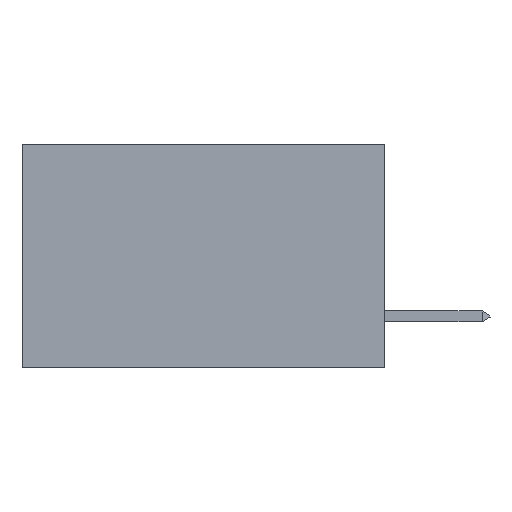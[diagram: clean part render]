
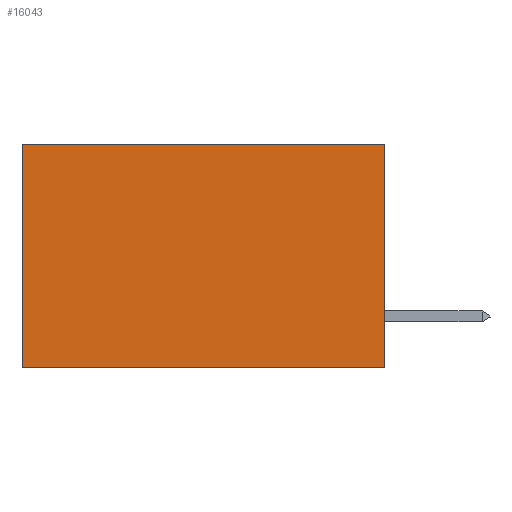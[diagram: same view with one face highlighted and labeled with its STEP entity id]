
A CAD part, left-side view. The second image highlights one B-rep face of the part: STEP entity #16043.
In plain terms, the highlighted planar face has unit normal (-1, 0, 0).
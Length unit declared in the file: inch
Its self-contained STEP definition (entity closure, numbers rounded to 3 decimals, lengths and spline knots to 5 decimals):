
#561 = EDGE_CURVE ( 'NONE', #37668, #39384, #48474, .T. ) ;
#1286 = DIRECTION ( 'NONE',  ( 0., 0., -1. ) ) ;
#5961 = CARTESIAN_POINT ( 'NONE',  ( 0.2875, 0., 0. ) ) ;
#7498 = VECTOR ( 'NONE', #41490, 39.37008 ) ;
#7872 = AXIS2_PLACEMENT_3D ( 'NONE', #12150, #24251, #1286 ) ;
#9865 = EDGE_CURVE ( 'NONE', #48452, #37668, #19689, .T. ) ;
#12098 = DIRECTION ( 'NONE',  ( 0., 1., 0. ) ) ;
#12150 = CARTESIAN_POINT ( 'NONE',  ( 0.2875, 0., 0. ) ) ;
#12496 = VECTOR ( 'NONE', #34595, 39.37008 ) ;
#13403 = DIRECTION ( 'NONE',  ( 0., 0., -1. ) ) ;
#13485 = EDGE_CURVE ( 'NONE', #48452, #42538, #37122, .T. ) ;
#14291 = VECTOR ( 'NONE', #13403, 39.37008 ) ;
#15569 = CARTESIAN_POINT ( 'NONE',  ( 0.2875, 0., 0. ) ) ;
#16043 = ADVANCED_FACE ( 'NONE', ( #45341 ), #35200, .F. ) ;
#18028 = ORIENTED_EDGE ( 'NONE', *, *, #24321, .T. ) ;
#18927 = CARTESIAN_POINT ( 'NONE',  ( 0.2875, 0.6, 0. ) ) ;
#19689 = LINE ( 'NONE', #5961, #14291 ) ;
#24251 = DIRECTION ( 'NONE',  ( 1., 0., 0. ) ) ;
#24321 = EDGE_CURVE ( 'NONE', #42538, #39384, #42543, .T. ) ;
#26009 = ORIENTED_EDGE ( 'NONE', *, *, #13485, .T. ) ;
#26875 = VECTOR ( 'NONE', #12098, 39.37008 ) ;
#29917 = CARTESIAN_POINT ( 'NONE',  ( 0.2875, 0., -0.37 ) ) ;
#30048 = ORIENTED_EDGE ( 'NONE', *, *, #561, .F. ) ;
#31444 = CARTESIAN_POINT ( 'NONE',  ( 0.2875, 0., 0. ) ) ;
#34595 = DIRECTION ( 'NONE',  ( 0., 0., -1. ) ) ;
#35200 = PLANE ( 'NONE',  #7872 ) ;
#36214 = CARTESIAN_POINT ( 'NONE',  ( 0.2875, 0.6, -0.37 ) ) ;
#36752 = EDGE_LOOP ( 'NONE', ( #18028, #30048, #45795, #26009 ) ) ;
#37122 = LINE ( 'NONE', #31444, #26875 ) ;
#37127 = CARTESIAN_POINT ( 'NONE',  ( 0.2875, 0., -0.37 ) ) ;
#37272 = CARTESIAN_POINT ( 'NONE',  ( 0.2875, 0.6, 0. ) ) ;
#37668 = VERTEX_POINT ( 'NONE', #29917 ) ;
#39384 = VERTEX_POINT ( 'NONE', #36214 ) ;
#41490 = DIRECTION ( 'NONE',  ( 0., 1., 0. ) ) ;
#42538 = VERTEX_POINT ( 'NONE', #37272 ) ;
#42543 = LINE ( 'NONE', #18927, #12496 ) ;
#45341 = FACE_OUTER_BOUND ( 'NONE', #36752, .T. ) ;
#45795 = ORIENTED_EDGE ( 'NONE', *, *, #9865, .F. ) ;
#48452 = VERTEX_POINT ( 'NONE', #15569 ) ;
#48474 = LINE ( 'NONE', #37127, #7498 ) ;
